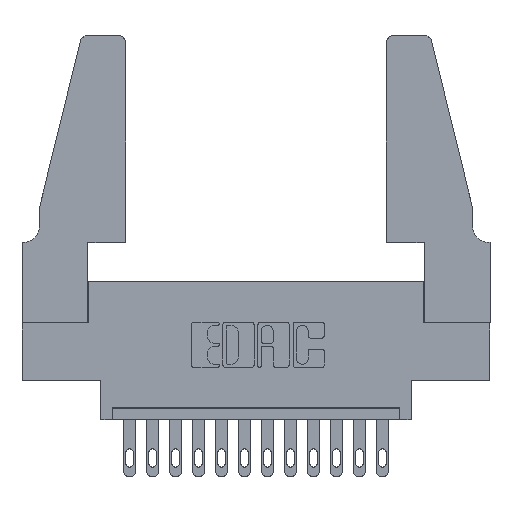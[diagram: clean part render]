
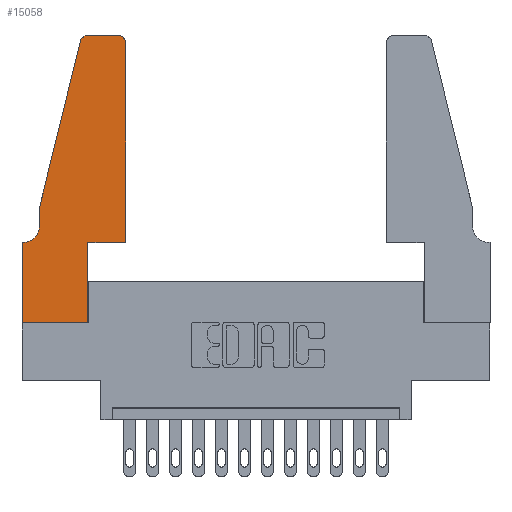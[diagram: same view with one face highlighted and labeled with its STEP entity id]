
A CAD part, top view. The second image highlights one B-rep face of the part: STEP entity #15058.
In plain terms, the highlighted planar face has unit normal (0, 0, 1).
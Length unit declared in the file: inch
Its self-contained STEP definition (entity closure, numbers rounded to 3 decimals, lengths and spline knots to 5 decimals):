
#105 = CARTESIAN_POINT ( 'NONE',  ( 0.284, 1.22, 0.37 ) ) ;
#184 = FACE_OUTER_BOUND ( 'NONE', #10554, .T. ) ;
#212 = DIRECTION ( 'NONE',  ( 1., 0., 0. ) ) ;
#348 = CARTESIAN_POINT ( 'NONE',  ( 0.0755, 0.42, 0.37 ) ) ;
#408 = CIRCLE ( 'NONE', #12530, 0.03 ) ;
#988 = CARTESIAN_POINT ( 'NONE',  ( 0.2865, 0.35, 0.37 ) ) ;
#1013 = DIRECTION ( 'NONE',  ( 0., -1., 0. ) ) ;
#1019 = ORIENTED_EDGE ( 'NONE', *, *, #1980, .T. ) ;
#1030 = ORIENTED_EDGE ( 'NONE', *, *, #12945, .T. ) ;
#1067 = VECTOR ( 'NONE', #1013, 39.37008 ) ;
#1137 = DIRECTION ( 'NONE',  ( 1., 0., 0. ) ) ;
#1226 = LINE ( 'NONE', #10439, #13073 ) ;
#1342 = DIRECTION ( 'NONE',  ( -0.239, -0.971, 0. ) ) ;
#1456 = DIRECTION ( 'NONE',  ( 0., 0., 1. ) ) ;
#1482 = VERTEX_POINT ( 'NONE', #2907 ) ;
#1703 = EDGE_CURVE ( 'NONE', #6912, #1482, #4423, .T. ) ;
#1976 = AXIS2_PLACEMENT_3D ( 'NONE', #10621, #2232, #1137 ) ;
#1980 = EDGE_CURVE ( 'NONE', #7662, #2688, #13606, .T. ) ;
#2232 = DIRECTION ( 'NONE',  ( 0., 0., 1. ) ) ;
#2365 = VERTEX_POINT ( 'NONE', #11240 ) ;
#2433 = ORIENTED_EDGE ( 'NONE', *, *, #14634, .T. ) ;
#2491 = DIRECTION ( 'NONE',  ( 0., 0., -1. ) ) ;
#2513 = ORIENTED_EDGE ( 'NONE', *, *, #13520, .T. ) ;
#2573 = LINE ( 'NONE', #10485, #13108 ) ;
#2688 = VERTEX_POINT ( 'NONE', #9454 ) ;
#2907 = CARTESIAN_POINT ( 'NONE',  ( 0.0055, 0.35, 0.37 ) ) ;
#3231 = LINE ( 'NONE', #988, #8392 ) ;
#3322 = EDGE_CURVE ( 'NONE', #9366, #10412, #408, .T. ) ;
#3395 = DIRECTION ( 'NONE',  ( 1., 0., 0. ) ) ;
#3546 = VERTEX_POINT ( 'NONE', #8015 ) ;
#3592 = DIRECTION ( 'NONE',  ( -1., 0., 0. ) ) ;
#3799 = VECTOR ( 'NONE', #10181, 39.37008 ) ;
#3983 = CARTESIAN_POINT ( 'NONE',  ( 0., 0., 0.37 ) ) ;
#4041 = EDGE_CURVE ( 'NONE', #14471, #9366, #5815, .T. ) ;
#4356 = DIRECTION ( 'NONE',  ( 0., 0., 1. ) ) ;
#4357 = VECTOR ( 'NONE', #3592, 39.37008 ) ;
#4423 = CIRCLE ( 'NONE', #15135, 0.07 ) ;
#4659 = DIRECTION ( 'NONE',  ( 0., 1., 0. ) ) ;
#4797 = CARTESIAN_POINT ( 'NONE',  ( 0.2865, 0.35, 0.37 ) ) ;
#5321 = AXIS2_PLACEMENT_3D ( 'NONE', #12483, #4356, #9025 ) ;
#5429 = CARTESIAN_POINT ( 'NONE',  ( 0.4505, 0.35, 0.37 ) ) ;
#5458 = EDGE_CURVE ( 'NONE', #10412, #2365, #2573, .T. ) ;
#5815 = LINE ( 'NONE', #10125, #3799 ) ;
#5981 = EDGE_CURVE ( 'NONE', #6643, #13330, #8692, .T. ) ;
#6421 = CARTESIAN_POINT ( 'NONE',  ( 0.284, 1.25, 0.37 ) ) ;
#6643 = VERTEX_POINT ( 'NONE', #5429 ) ;
#6788 = CARTESIAN_POINT ( 'NONE',  ( 0.0755, 0.5, 0.37 ) ) ;
#6912 = VERTEX_POINT ( 'NONE', #348 ) ;
#6965 = ORIENTED_EDGE ( 'NONE', *, *, #5458, .T. ) ;
#7039 = CARTESIAN_POINT ( 'NONE',  ( 0.0755, 0.35, 0.37 ) ) ;
#7063 = ORIENTED_EDGE ( 'NONE', *, *, #1703, .T. ) ;
#7276 = CARTESIAN_POINT ( 'NONE',  ( 0.0055, 0.42, 0.37 ) ) ;
#7311 = VECTOR ( 'NONE', #11524, 39.37008 ) ;
#7603 = EDGE_CURVE ( 'NONE', #10751, #6643, #1226, .T. ) ;
#7662 = VERTEX_POINT ( 'NONE', #12951 ) ;
#8015 = CARTESIAN_POINT ( 'NONE',  ( 0.2865, 0., 0.37 ) ) ;
#8392 = VECTOR ( 'NONE', #4659, 39.37008 ) ;
#8692 = LINE ( 'NONE', #11791, #11091 ) ;
#9025 = DIRECTION ( 'NONE',  ( 1., 0., 0. ) ) ;
#9282 = ORIENTED_EDGE ( 'NONE', *, *, #10963, .T. ) ;
#9366 = VERTEX_POINT ( 'NONE', #6421 ) ;
#9454 = CARTESIAN_POINT ( 'NONE',  ( 0., 0., 0.37 ) ) ;
#9629 = ORIENTED_EDGE ( 'NONE', *, *, #7603, .T. ) ;
#9635 = ORIENTED_EDGE ( 'NONE', *, *, #3322, .T. ) ;
#10115 = VECTOR ( 'NONE', #14641, 39.37008 ) ;
#10125 = CARTESIAN_POINT ( 'NONE',  ( 0.2605, 1.25, 0.37 ) ) ;
#10181 = DIRECTION ( 'NONE',  ( -1., 0., 0. ) ) ;
#10257 = LINE ( 'NONE', #10262, #7311 ) ;
#10262 = CARTESIAN_POINT ( 'NONE',  ( 0., 0., 0.37 ) ) ;
#10300 = PLANE ( 'NONE',  #5321 ) ;
#10412 = VERTEX_POINT ( 'NONE', #14016 ) ;
#10439 = CARTESIAN_POINT ( 'NONE',  ( 0.4505, 0.35, 0.37 ) ) ;
#10481 = CARTESIAN_POINT ( 'NONE',  ( 0.4205, 1.25, 0.37 ) ) ;
#10485 = CARTESIAN_POINT ( 'NONE',  ( 0.0755, 0.5, 0.37 ) ) ;
#10554 = EDGE_LOOP ( 'NONE', ( #14858, #9635, #6965, #13140, #7063, #2433, #1019, #1030, #2513, #9629, #14512, #9282 ) ) ;
#10605 = LINE ( 'NONE', #7039, #4357 ) ;
#10621 = CARTESIAN_POINT ( 'NONE',  ( 0.4205, 1.22, 0.37 ) ) ;
#10648 = EDGE_CURVE ( 'NONE', #2365, #6912, #12738, .T. ) ;
#10676 = DIRECTION ( 'NONE',  ( -1., 0., 0. ) ) ;
#10751 = VERTEX_POINT ( 'NONE', #4797 ) ;
#10963 = EDGE_CURVE ( 'NONE', #13330, #14471, #14194, .T. ) ;
#11091 = VECTOR ( 'NONE', #13181, 39.37008 ) ;
#11140 = CARTESIAN_POINT ( 'NONE',  ( 0.4505, 1.22, 0.37 ) ) ;
#11240 = CARTESIAN_POINT ( 'NONE',  ( 0.0755, 0.5, 0.37 ) ) ;
#11524 = DIRECTION ( 'NONE',  ( 1., 0., 0. ) ) ;
#11791 = CARTESIAN_POINT ( 'NONE',  ( 0.4505, 0.35, 0.37 ) ) ;
#12483 = CARTESIAN_POINT ( 'NONE',  ( 0., 0.35, 0.37 ) ) ;
#12530 = AXIS2_PLACEMENT_3D ( 'NONE', #105, #1456, #212 ) ;
#12738 = LINE ( 'NONE', #6788, #1067 ) ;
#12945 = EDGE_CURVE ( 'NONE', #2688, #3546, #10257, .T. ) ;
#12951 = CARTESIAN_POINT ( 'NONE',  ( 0., 0.35, 0.37 ) ) ;
#13073 = VECTOR ( 'NONE', #3395, 39.37008 ) ;
#13108 = VECTOR ( 'NONE', #1342, 39.37008 ) ;
#13140 = ORIENTED_EDGE ( 'NONE', *, *, #10648, .T. ) ;
#13181 = DIRECTION ( 'NONE',  ( 0., 1., 0. ) ) ;
#13330 = VERTEX_POINT ( 'NONE', #11140 ) ;
#13520 = EDGE_CURVE ( 'NONE', #3546, #10751, #3231, .T. ) ;
#13606 = LINE ( 'NONE', #3983, #10115 ) ;
#14016 = CARTESIAN_POINT ( 'NONE',  ( 0.25487, 1.22718, 0.37 ) ) ;
#14194 = CIRCLE ( 'NONE', #1976, 0.03 ) ;
#14471 = VERTEX_POINT ( 'NONE', #10481 ) ;
#14512 = ORIENTED_EDGE ( 'NONE', *, *, #5981, .T. ) ;
#14634 = EDGE_CURVE ( 'NONE', #1482, #7662, #10605, .T. ) ;
#14641 = DIRECTION ( 'NONE',  ( 0., -1., 0. ) ) ;
#14858 = ORIENTED_EDGE ( 'NONE', *, *, #4041, .T. ) ;
#15058 = ADVANCED_FACE ( 'NONE', ( #184 ), #10300, .T. ) ;
#15135 = AXIS2_PLACEMENT_3D ( 'NONE', #7276, #2491, #10676 ) ;
